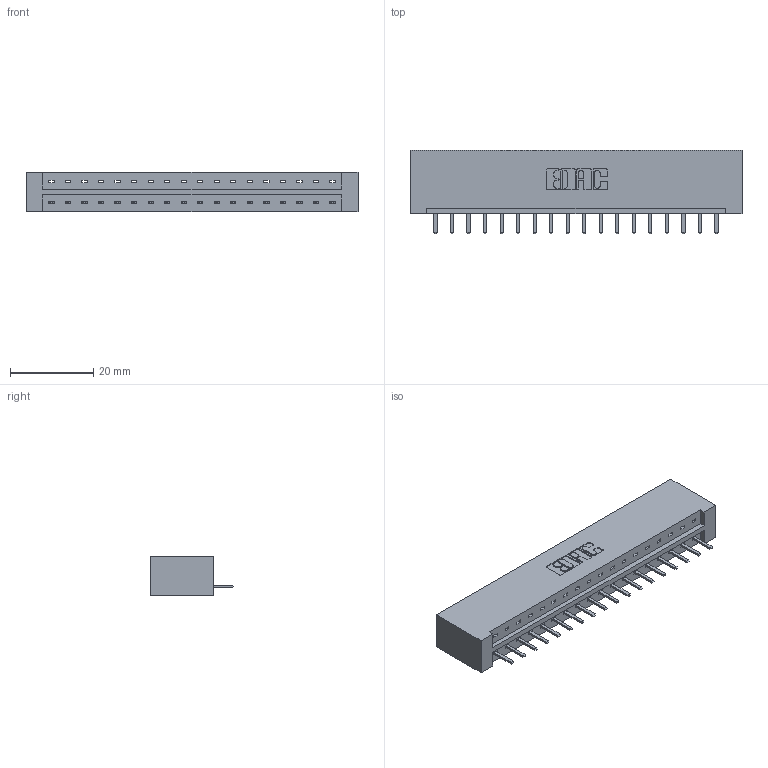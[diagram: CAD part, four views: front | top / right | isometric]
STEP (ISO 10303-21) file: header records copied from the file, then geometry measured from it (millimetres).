
FILE_DESCRIPTION (( 'STEP AP203' ), '1' );
FILE_NAME ('333-018-520-101.STEP', '2019-08-09T12:37:13', ( '' ), ( '' ), 'SwSTEP 2.0', 'SolidWorks 2016', '' );
FILE_SCHEMA (( 'CONFIG_CONTROL_DESIGN' ));
Length unit declared in the file: inch
Products named in the file (3): 345-292-001_345-293-120; 333 Part_Lugless; 333-018-520-101
Assembly tree (19 placements, depth 2):
  333-018-520-101
    333 Part_Lugless
    345-292-001_345-293-120  x18
Bounding box: 79.58 x 20.02 x 9.4 mm (x, y, z)
Volume: 8362.4 mm3; surface area: 8665.7 mm2
Topology: 19 solids, 19 shells, 1222 faces, 3599 edges, 2350 vertices
Faces by surface type: plane 858, cylinder 364
Entity records: 13945 total; most frequent: CARTESIAN_POINT 2428, ORIENTED_EDGE 2370, DIRECTION 2077, EDGE_CURVE 1185, LINE 1061, VECTOR 1061, VERTEX_POINT 786, AXIS2_PLACEMENT_3D 508
